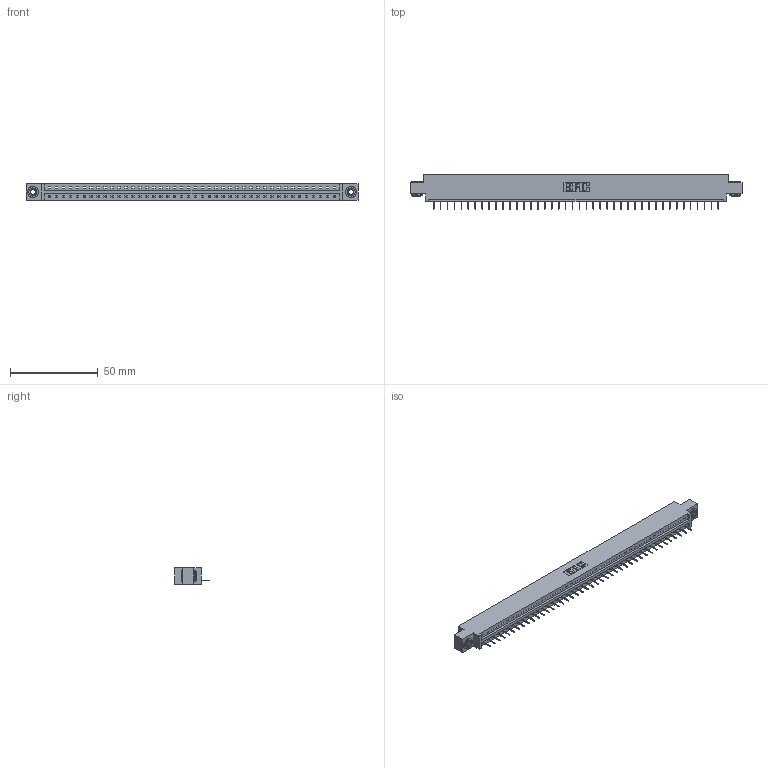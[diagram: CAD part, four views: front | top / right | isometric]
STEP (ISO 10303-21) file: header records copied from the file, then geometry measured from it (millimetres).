
FILE_DESCRIPTION (( 'STEP AP203' ), '1' );
FILE_NAME ('337-042-524-603.STEP', '2019-10-01T22:03:34', ( '' ), ( '' ), 'SwSTEP 2.0', 'SolidWorks 2016', '' );
FILE_SCHEMA (( 'CONFIG_CONTROL_DESIGN' ));
Length unit declared in the file: inch
Products named in the file (4): 337 Part_0.170 Offset - 0.156 Dia-TH; 345-250-002_345-250-002-102; 337-042-524-603; 345-292-001_345-293-124
Assembly tree (45 placements, depth 2):
  337-042-524-603
    337 Part_0.170 Offset - 0.156 Dia-TH
    345-292-001_345-293-124  x42
    345-250-002_345-250-002-102  x2
Bounding box: 189.43 x 19.69 x 9.4 mm (x, y, z)
Volume: 19424.4 mm3; surface area: 19817.9 mm2
Topology: 45 solids, 45 shells, 2928 faces, 8463 edges, 5470 vertices
Faces by surface type: plane 2268, cylinder 652, cone 8
Entity records: 32076 total; most frequent: CARTESIAN_POINT 5563, ORIENTED_EDGE 5534, DIRECTION 4717, EDGE_CURVE 2767, VECTOR 2619, LINE 2619, VERTEX_POINT 1838, AXIS2_PLACEMENT_3D 1049
